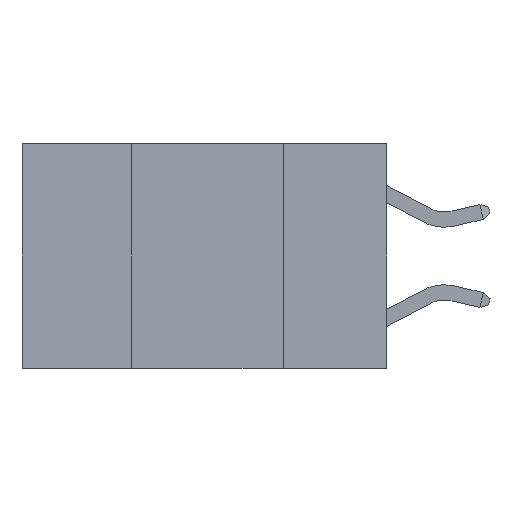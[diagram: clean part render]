
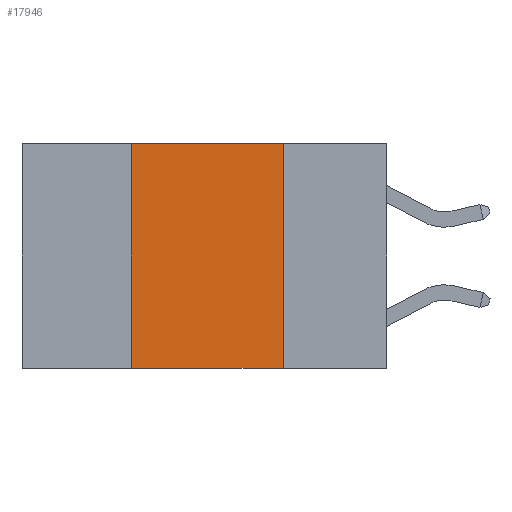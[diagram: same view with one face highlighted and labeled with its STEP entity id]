
A CAD part, left-side view. The second image highlights one B-rep face of the part: STEP entity #17946.
In plain terms, the highlighted planar face has unit normal (-1, 0, 0).
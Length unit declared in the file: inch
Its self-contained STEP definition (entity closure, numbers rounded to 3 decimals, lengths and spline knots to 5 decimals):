
#817 = VECTOR ( 'NONE', #9751, 39.37008 ) ;
#1121 = VERTEX_POINT ( 'NONE', #8563 ) ;
#1139 = CARTESIAN_POINT ( 'NONE',  ( 0., 0.6, 0. ) ) ;
#1226 = DIRECTION ( 'NONE',  ( 0., 0., -1. ) ) ;
#1704 = LINE ( 'NONE', #11850, #4183 ) ;
#2106 = EDGE_CURVE ( 'NONE', #1121, #11112, #1704, .T. ) ;
#2365 = ORIENTED_EDGE ( 'NONE', *, *, #2106, .T. ) ;
#2870 = VERTEX_POINT ( 'NONE', #14224 ) ;
#4183 = VECTOR ( 'NONE', #7394, 39.37008 ) ;
#5103 = AXIS2_PLACEMENT_3D ( 'NONE', #1139, #12023, #1226 ) ;
#5555 = ORIENTED_EDGE ( 'NONE', *, *, #6417, .F. ) ;
#5861 = EDGE_CURVE ( 'NONE', #2870, #11112, #7274, .T. ) ;
#5892 = VECTOR ( 'NONE', #11952, 39.37008 ) ;
#6417 = EDGE_CURVE ( 'NONE', #1121, #17968, #13364, .T. ) ;
#7274 = LINE ( 'NONE', #16840, #13009 ) ;
#7394 = DIRECTION ( 'NONE',  ( 0., -1., 0. ) ) ;
#7860 = CARTESIAN_POINT ( 'NONE',  ( 0., 0.42, 0. ) ) ;
#8308 = DIRECTION ( 'NONE',  ( 0., 0., -1. ) ) ;
#8563 = CARTESIAN_POINT ( 'NONE',  ( 0., 0.42, -0.37 ) ) ;
#9050 = EDGE_LOOP ( 'NONE', ( #14696, #14238, #5555, #2365 ) ) ;
#9605 = FACE_OUTER_BOUND ( 'NONE', #9050, .T. ) ;
#9751 = DIRECTION ( 'NONE',  ( 0., -1., 0. ) ) ;
#11112 = VERTEX_POINT ( 'NONE', #18330 ) ;
#11527 = EDGE_CURVE ( 'NONE', #17968, #2870, #14409, .T. ) ;
#11850 = CARTESIAN_POINT ( 'NONE',  ( 0., 0.6, -0.37 ) ) ;
#11952 = DIRECTION ( 'NONE',  ( 0., 0., 1. ) ) ;
#12023 = DIRECTION ( 'NONE',  ( 1., 0., 0. ) ) ;
#13009 = VECTOR ( 'NONE', #8308, 39.37008 ) ;
#13364 = LINE ( 'NONE', #7860, #5892 ) ;
#13902 = PLANE ( 'NONE',  #5103 ) ;
#14224 = CARTESIAN_POINT ( 'NONE',  ( 0., 0.17, 0. ) ) ;
#14232 = CARTESIAN_POINT ( 'NONE',  ( 0., 0.6, 0. ) ) ;
#14238 = ORIENTED_EDGE ( 'NONE', *, *, #11527, .F. ) ;
#14409 = LINE ( 'NONE', #14232, #817 ) ;
#14696 = ORIENTED_EDGE ( 'NONE', *, *, #5861, .F. ) ;
#16840 = CARTESIAN_POINT ( 'NONE',  ( 0., 0.17, 0. ) ) ;
#16942 = CARTESIAN_POINT ( 'NONE',  ( 0., 0.42, 0. ) ) ;
#17946 = ADVANCED_FACE ( 'NONE', ( #9605 ), #13902, .F. ) ;
#17968 = VERTEX_POINT ( 'NONE', #16942 ) ;
#18330 = CARTESIAN_POINT ( 'NONE',  ( 0., 0.17, -0.37 ) ) ;
